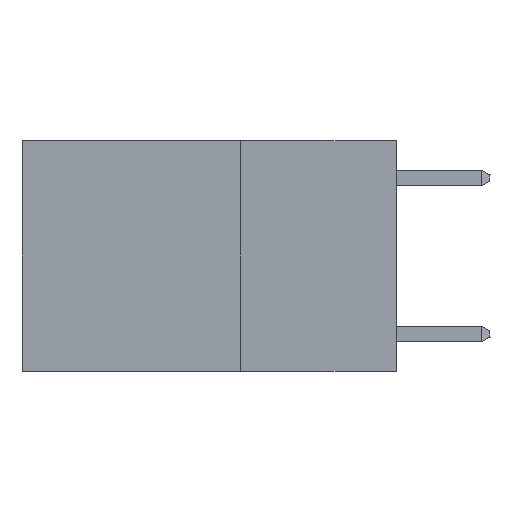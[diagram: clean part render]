
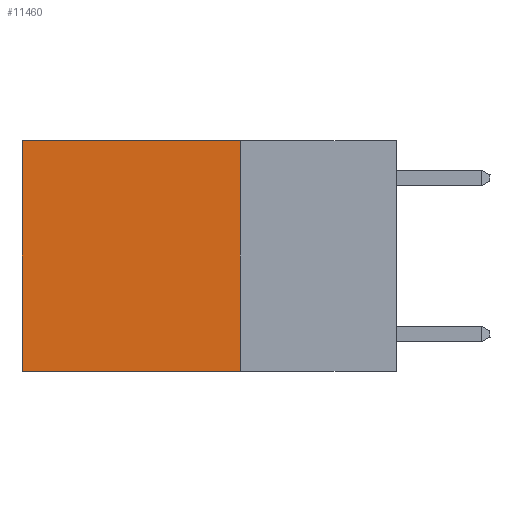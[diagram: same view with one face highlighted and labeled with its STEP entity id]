
A CAD part, left-side view. The second image highlights one B-rep face of the part: STEP entity #11460.
In plain terms, the highlighted planar face has unit normal (-1, 0, 0).
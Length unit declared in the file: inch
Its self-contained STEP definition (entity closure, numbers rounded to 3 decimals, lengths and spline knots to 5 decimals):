
#4 = CARTESIAN_POINT ( 'NONE',  ( 0.2625, 0.25, 0. ) ) ;
#783 = ORIENTED_EDGE ( 'NONE', *, *, #24682, .F. ) ;
#980 = CARTESIAN_POINT ( 'NONE',  ( 0.2625, 0.25, -0.37 ) ) ;
#1679 = VERTEX_POINT ( 'NONE', #25026 ) ;
#1743 = ORIENTED_EDGE ( 'NONE', *, *, #1882, .T. ) ;
#1882 = EDGE_CURVE ( 'NONE', #4315, #4078, #19260, .T. ) ;
#3285 = DIRECTION ( 'NONE',  ( 0., 1., 0. ) ) ;
#3711 = CARTESIAN_POINT ( 'NONE',  ( 0.2625, 0.6, -0.37 ) ) ;
#4078 = VERTEX_POINT ( 'NONE', #3711 ) ;
#4315 = VERTEX_POINT ( 'NONE', #24152 ) ;
#4788 = CARTESIAN_POINT ( 'NONE',  ( 0.2625, 0.25, -0.37 ) ) ;
#4973 = LINE ( 'NONE', #5102, #8529 ) ;
#5102 = CARTESIAN_POINT ( 'NONE',  ( 0.2625, 0.25, 0. ) ) ;
#5994 = ORIENTED_EDGE ( 'NONE', *, *, #12190, .F. ) ;
#6369 = EDGE_LOOP ( 'NONE', ( #1743, #5994, #783, #7234 ) ) ;
#6658 = EDGE_CURVE ( 'NONE', #1679, #4315, #22879, .T. ) ;
#7234 = ORIENTED_EDGE ( 'NONE', *, *, #6658, .T. ) ;
#7444 = DIRECTION ( 'NONE',  ( 1., 0., 0. ) ) ;
#7873 = AXIS2_PLACEMENT_3D ( 'NONE', #4, #7444, #17292 ) ;
#7999 = CARTESIAN_POINT ( 'NONE',  ( 0.2625, 0.6, 0. ) ) ;
#8529 = VECTOR ( 'NONE', #16356, 39.37008 ) ;
#10662 = VERTEX_POINT ( 'NONE', #4788 ) ;
#11460 = ADVANCED_FACE ( 'NONE', ( #22926 ), #17671, .F. ) ;
#12190 = EDGE_CURVE ( 'NONE', #10662, #4078, #12738, .T. ) ;
#12738 = LINE ( 'NONE', #980, #17353 ) ;
#13997 = VECTOR ( 'NONE', #15794, 39.37008 ) ;
#15794 = DIRECTION ( 'NONE',  ( 0., 0., -1. ) ) ;
#16356 = DIRECTION ( 'NONE',  ( 0., 0., -1. ) ) ;
#16910 = VECTOR ( 'NONE', #3285, 39.37008 ) ;
#17292 = DIRECTION ( 'NONE',  ( 0., 0., -1. ) ) ;
#17353 = VECTOR ( 'NONE', #24661, 39.37008 ) ;
#17671 = PLANE ( 'NONE',  #7873 ) ;
#19260 = LINE ( 'NONE', #7999, #13997 ) ;
#20843 = CARTESIAN_POINT ( 'NONE',  ( 0.2625, 0.25, 0. ) ) ;
#22879 = LINE ( 'NONE', #20843, #16910 ) ;
#22926 = FACE_OUTER_BOUND ( 'NONE', #6369, .T. ) ;
#24152 = CARTESIAN_POINT ( 'NONE',  ( 0.2625, 0.6, 0. ) ) ;
#24661 = DIRECTION ( 'NONE',  ( 0., 1., 0. ) ) ;
#24682 = EDGE_CURVE ( 'NONE', #1679, #10662, #4973, .T. ) ;
#25026 = CARTESIAN_POINT ( 'NONE',  ( 0.2625, 0.25, 0. ) ) ;
